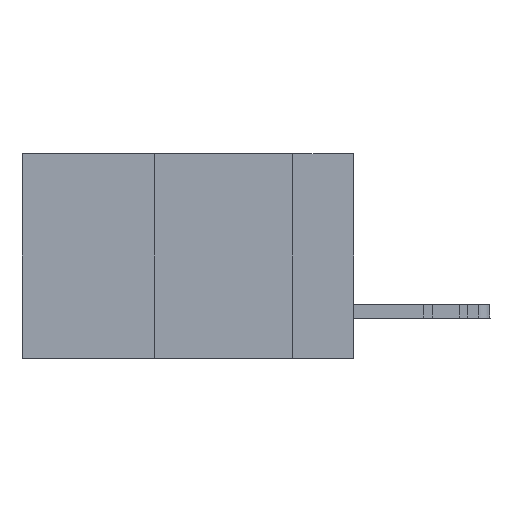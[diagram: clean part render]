
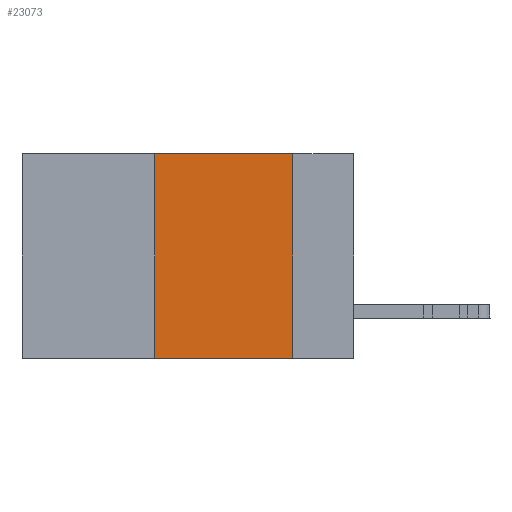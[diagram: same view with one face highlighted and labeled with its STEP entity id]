
A CAD part, left-side view. The second image highlights one B-rep face of the part: STEP entity #23073.
In plain terms, the highlighted planar face has unit normal (-1, 0, 0).
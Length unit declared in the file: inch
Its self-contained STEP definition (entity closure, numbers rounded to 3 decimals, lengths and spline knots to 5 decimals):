
#361 = VECTOR ( 'NONE', #22565, 39.37008 ) ;
#1918 = CARTESIAN_POINT ( 'NONE',  ( 0., 0.11, -0.37 ) ) ;
#2279 = EDGE_LOOP ( 'NONE', ( #38592, #19565, #26571, #33845 ) ) ;
#4322 = EDGE_CURVE ( 'NONE', #24727, #40052, #21827, .T. ) ;
#6043 = VERTEX_POINT ( 'NONE', #13821 ) ;
#6812 = LINE ( 'NONE', #36166, #39020 ) ;
#6999 = FACE_OUTER_BOUND ( 'NONE', #2279, .T. ) ;
#7430 = VERTEX_POINT ( 'NONE', #1918 ) ;
#8898 = EDGE_CURVE ( 'NONE', #6043, #7430, #10191, .T. ) ;
#9150 = AXIS2_PLACEMENT_3D ( 'NONE', #14839, #35646, #28664 ) ;
#10191 = LINE ( 'NONE', #25418, #37522 ) ;
#12055 = EDGE_CURVE ( 'NONE', #40052, #6043, #13328, .T. ) ;
#13035 = CARTESIAN_POINT ( 'NONE',  ( 0., 0.36, 0. ) ) ;
#13328 = LINE ( 'NONE', #36287, #15745 ) ;
#13821 = CARTESIAN_POINT ( 'NONE',  ( 0., 0.11, 0. ) ) ;
#13888 = EDGE_CURVE ( 'NONE', #24727, #7430, #6812, .T. ) ;
#14839 = CARTESIAN_POINT ( 'NONE',  ( 0., 0.6, 0. ) ) ;
#15745 = VECTOR ( 'NONE', #21094, 39.37008 ) ;
#19371 = CARTESIAN_POINT ( 'NONE',  ( 0., 0.36, 0. ) ) ;
#19565 = ORIENTED_EDGE ( 'NONE', *, *, #12055, .F. ) ;
#21094 = DIRECTION ( 'NONE',  ( 0., -1., 0. ) ) ;
#21827 = LINE ( 'NONE', #13035, #361 ) ;
#22565 = DIRECTION ( 'NONE',  ( 0., 0., 1. ) ) ;
#22834 = PLANE ( 'NONE',  #9150 ) ;
#23073 = ADVANCED_FACE ( 'NONE', ( #6999 ), #22834, .F. ) ;
#24727 = VERTEX_POINT ( 'NONE', #25122 ) ;
#25122 = CARTESIAN_POINT ( 'NONE',  ( 0., 0.36, -0.37 ) ) ;
#25418 = CARTESIAN_POINT ( 'NONE',  ( 0., 0.11, 0. ) ) ;
#26571 = ORIENTED_EDGE ( 'NONE', *, *, #4322, .F. ) ;
#28664 = DIRECTION ( 'NONE',  ( 0., 0., -1. ) ) ;
#33845 = ORIENTED_EDGE ( 'NONE', *, *, #13888, .T. ) ;
#34052 = DIRECTION ( 'NONE',  ( 0., -1., 0. ) ) ;
#35118 = DIRECTION ( 'NONE',  ( 0., 0., -1. ) ) ;
#35646 = DIRECTION ( 'NONE',  ( 1., 0., 0. ) ) ;
#36166 = CARTESIAN_POINT ( 'NONE',  ( 0., 0.6, -0.37 ) ) ;
#36287 = CARTESIAN_POINT ( 'NONE',  ( 0., 0.6, 0. ) ) ;
#37522 = VECTOR ( 'NONE', #35118, 39.37008 ) ;
#38592 = ORIENTED_EDGE ( 'NONE', *, *, #8898, .F. ) ;
#39020 = VECTOR ( 'NONE', #34052, 39.37008 ) ;
#40052 = VERTEX_POINT ( 'NONE', #19371 ) ;
